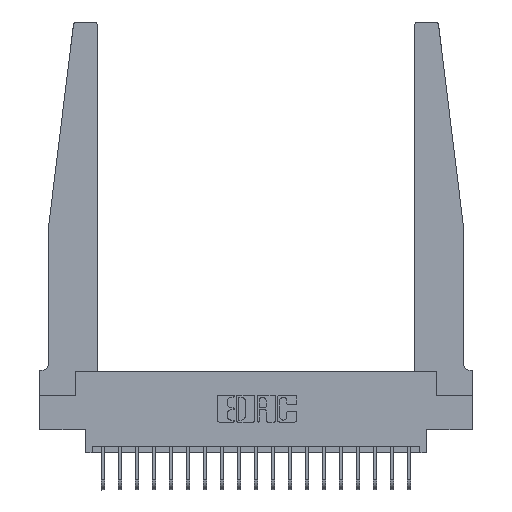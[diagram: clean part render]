
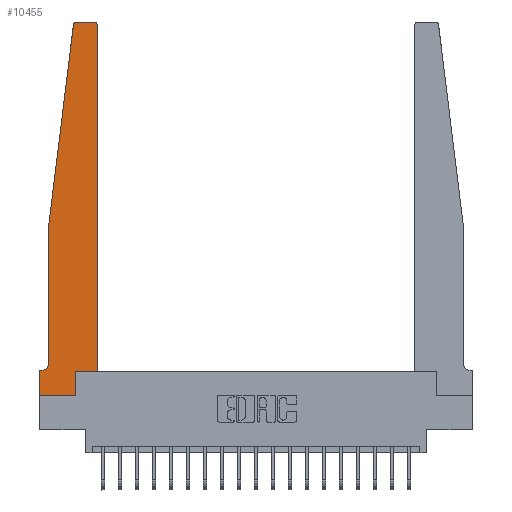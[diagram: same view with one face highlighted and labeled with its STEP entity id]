
A CAD part, top view. The second image highlights one B-rep face of the part: STEP entity #10455.
In plain terms, the highlighted planar face has unit normal (0, 0, 1).
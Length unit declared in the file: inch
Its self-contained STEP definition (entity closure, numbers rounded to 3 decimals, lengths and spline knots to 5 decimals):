
#16 = DIRECTION ( 'NONE',  ( 0., 0., 1. ) ) ;
#66 = VERTEX_POINT ( 'NONE', #5508 ) ;
#727 = DIRECTION ( 'NONE',  ( 0., 0., -1. ) ) ;
#790 = CARTESIAN_POINT ( 'NONE',  ( 0.425, 0.18, 0.37 ) ) ;
#889 = ORIENTED_EDGE ( 'NONE', *, *, #5272, .T. ) ;
#966 = DIRECTION ( 'NONE',  ( 0., 0., 1. ) ) ;
#1033 = EDGE_CURVE ( 'NONE', #16785, #8592, #16869, .T. ) ;
#1058 = EDGE_CURVE ( 'NONE', #4223, #16719, #4717, .T. ) ;
#1208 = VECTOR ( 'NONE', #15903, 39.37008 ) ;
#1403 = AXIS2_PLACEMENT_3D ( 'NONE', #10066, #727, #11604 ) ;
#1508 = CARTESIAN_POINT ( 'NONE',  ( 0., 0., 0.37 ) ) ;
#1582 = CARTESIAN_POINT ( 'NONE',  ( 0.2605, 0.18, 0.37 ) ) ;
#1768 = LINE ( 'NONE', #17251, #13152 ) ;
#1870 = DIRECTION ( 'NONE',  ( 0., -1., 0. ) ) ;
#1934 = CARTESIAN_POINT ( 'NONE',  ( 0.2605, 0.18, 0.37 ) ) ;
#2210 = CARTESIAN_POINT ( 'NONE',  ( 0.27653, 2.75, 0.37 ) ) ;
#2229 = EDGE_CURVE ( 'NONE', #8592, #66, #17530, .T. ) ;
#2535 = ORIENTED_EDGE ( 'NONE', *, *, #4785, .T. ) ;
#2541 = LINE ( 'NONE', #12716, #14359 ) ;
#3466 = DIRECTION ( 'NONE',  ( 0., 1., 0. ) ) ;
#3479 = PLANE ( 'NONE',  #8309 ) ;
#3625 = CARTESIAN_POINT ( 'NONE',  ( 0.25, 2.75, 0.37 ) ) ;
#3840 = CARTESIAN_POINT ( 'NONE',  ( 0.425, 0.18, 0.37 ) ) ;
#4073 = AXIS2_PLACEMENT_3D ( 'NONE', #9398, #16, #10921 ) ;
#4101 = ORIENTED_EDGE ( 'NONE', *, *, #2229, .T. ) ;
#4223 = VERTEX_POINT ( 'NONE', #1934 ) ;
#4231 = VECTOR ( 'NONE', #15082, 39.37008 ) ;
#4306 = VERTEX_POINT ( 'NONE', #10022 ) ;
#4537 = CARTESIAN_POINT ( 'NONE',  ( 0.24675, 2.72367, 0.37 ) ) ;
#4717 = LINE ( 'NONE', #790, #8391 ) ;
#4785 = EDGE_CURVE ( 'NONE', #4306, #9950, #18615, .T. ) ;
#4788 = EDGE_CURVE ( 'NONE', #66, #10303, #10591, .T. ) ;
#5077 = LINE ( 'NONE', #1582, #12770 ) ;
#5111 = DIRECTION ( 'NONE',  ( 0., 0., 1. ) ) ;
#5243 = DIRECTION ( 'NONE',  ( -1., 0., 0. ) ) ;
#5272 = EDGE_CURVE ( 'NONE', #9950, #16997, #14124, .T. ) ;
#5508 = CARTESIAN_POINT ( 'NONE',  ( 0., 0.1875, 0.37 ) ) ;
#6051 = EDGE_CURVE ( 'NONE', #19372, #16785, #2541, .T. ) ;
#6213 = CARTESIAN_POINT ( 'NONE',  ( 0., 0., 0.37 ) ) ;
#6556 = VECTOR ( 'NONE', #5243, 39.37008 ) ;
#7256 = VECTOR ( 'NONE', #16798, 39.37008 ) ;
#7782 = FACE_OUTER_BOUND ( 'NONE', #9049, .T. ) ;
#8309 = AXIS2_PLACEMENT_3D ( 'NONE', #14256, #5111, #15759 ) ;
#8391 = VECTOR ( 'NONE', #11667, 39.37008 ) ;
#8397 = CIRCLE ( 'NONE', #15201, 0.03 ) ;
#8592 = VERTEX_POINT ( 'NONE', #9256 ) ;
#9049 = EDGE_LOOP ( 'NONE', ( #2535, #889, #15525, #16458, #12893, #4101, #17224, #15616, #10000, #10943, #10495, #11093 ) ) ;
#9256 = CARTESIAN_POINT ( 'NONE',  ( 0.015, 0.1875, 0.37 ) ) ;
#9398 = CARTESIAN_POINT ( 'NONE',  ( 0.27653, 2.72, 0.37 ) ) ;
#9950 = VERTEX_POINT ( 'NONE', #2210 ) ;
#10000 = ORIENTED_EDGE ( 'NONE', *, *, #10338, .T. ) ;
#10022 = CARTESIAN_POINT ( 'NONE',  ( 0.395, 2.75, 0.37 ) ) ;
#10066 = CARTESIAN_POINT ( 'NONE',  ( 0.015, 0.2375, 0.37 ) ) ;
#10293 = CARTESIAN_POINT ( 'NONE',  ( 0.395, 2.72, 0.37 ) ) ;
#10303 = VERTEX_POINT ( 'NONE', #1508 ) ;
#10338 = EDGE_CURVE ( 'NONE', #15237, #4223, #5077, .T. ) ;
#10455 = ADVANCED_FACE ( 'NONE', ( #7782 ), #3479, .T. ) ;
#10495 = ORIENTED_EDGE ( 'NONE', *, *, #12258, .T. ) ;
#10591 = LINE ( 'NONE', #15892, #18150 ) ;
#10912 = EDGE_CURVE ( 'NONE', #10303, #15237, #15776, .T. ) ;
#10921 = DIRECTION ( 'NONE',  ( 1., 0., 0. ) ) ;
#10943 = ORIENTED_EDGE ( 'NONE', *, *, #1058, .T. ) ;
#11093 = ORIENTED_EDGE ( 'NONE', *, *, #17868, .T. ) ;
#11604 = DIRECTION ( 'NONE',  ( -1., 0., 0. ) ) ;
#11667 = DIRECTION ( 'NONE',  ( 1., 0., 0. ) ) ;
#11842 = DIRECTION ( 'NONE',  ( 1., 0., 0. ) ) ;
#12258 = EDGE_CURVE ( 'NONE', #16719, #16604, #1768, .T. ) ;
#12544 = EDGE_CURVE ( 'NONE', #16997, #19372, #16403, .T. ) ;
#12716 = CARTESIAN_POINT ( 'NONE',  ( 0.065, 1.25, 0.37 ) ) ;
#12770 = VECTOR ( 'NONE', #13990, 39.37008 ) ;
#12893 = ORIENTED_EDGE ( 'NONE', *, *, #1033, .T. ) ;
#13152 = VECTOR ( 'NONE', #3466, 39.37008 ) ;
#13990 = DIRECTION ( 'NONE',  ( 0., 1., 0. ) ) ;
#14124 = CIRCLE ( 'NONE', #4073, 0.03 ) ;
#14256 = CARTESIAN_POINT ( 'NONE',  ( 0., 0.1875, 0.37 ) ) ;
#14359 = VECTOR ( 'NONE', #1870, 39.37008 ) ;
#15082 = DIRECTION ( 'NONE',  ( -0.122, -0.992, 0. ) ) ;
#15201 = AXIS2_PLACEMENT_3D ( 'NONE', #10293, #966, #11842 ) ;
#15237 = VERTEX_POINT ( 'NONE', #17587 ) ;
#15525 = ORIENTED_EDGE ( 'NONE', *, *, #12544, .T. ) ;
#15616 = ORIENTED_EDGE ( 'NONE', *, *, #10912, .T. ) ;
#15759 = DIRECTION ( 'NONE',  ( 1., 0., 0. ) ) ;
#15776 = LINE ( 'NONE', #6213, #7256 ) ;
#15892 = CARTESIAN_POINT ( 'NONE',  ( 0., 0., 0.37 ) ) ;
#15903 = DIRECTION ( 'NONE',  ( -1., 0., 0. ) ) ;
#16403 = LINE ( 'NONE', #18093, #4231 ) ;
#16458 = ORIENTED_EDGE ( 'NONE', *, *, #6051, .T. ) ;
#16604 = VERTEX_POINT ( 'NONE', #17138 ) ;
#16719 = VERTEX_POINT ( 'NONE', #3840 ) ;
#16785 = VERTEX_POINT ( 'NONE', #19171 ) ;
#16798 = DIRECTION ( 'NONE',  ( 1., 0., 0. ) ) ;
#16869 = CIRCLE ( 'NONE', #1403, 0.05 ) ;
#16997 = VERTEX_POINT ( 'NONE', #4537 ) ;
#17138 = CARTESIAN_POINT ( 'NONE',  ( 0.425, 2.72, 0.37 ) ) ;
#17224 = ORIENTED_EDGE ( 'NONE', *, *, #4788, .T. ) ;
#17251 = CARTESIAN_POINT ( 'NONE',  ( 0.425, 0.18, 0.37 ) ) ;
#17393 = DIRECTION ( 'NONE',  ( 0., -1., 0. ) ) ;
#17530 = LINE ( 'NONE', #18923, #1208 ) ;
#17587 = CARTESIAN_POINT ( 'NONE',  ( 0.2605, 0., 0.37 ) ) ;
#17868 = EDGE_CURVE ( 'NONE', #16604, #4306, #8397, .T. ) ;
#18093 = CARTESIAN_POINT ( 'NONE',  ( 0.065, 1.25, 0.37 ) ) ;
#18150 = VECTOR ( 'NONE', #17393, 39.37008 ) ;
#18615 = LINE ( 'NONE', #3625, #6556 ) ;
#18923 = CARTESIAN_POINT ( 'NONE',  ( 0.065, 0.1875, 0.37 ) ) ;
#18938 = CARTESIAN_POINT ( 'NONE',  ( 0.065, 1.25, 0.37 ) ) ;
#19171 = CARTESIAN_POINT ( 'NONE',  ( 0.065, 0.2375, 0.37 ) ) ;
#19372 = VERTEX_POINT ( 'NONE', #18938 ) ;
